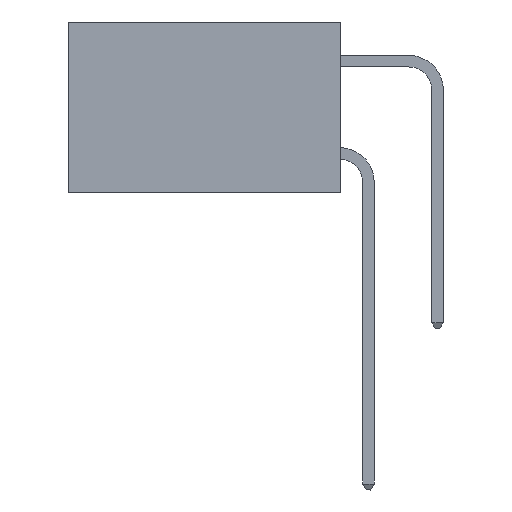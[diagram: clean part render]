
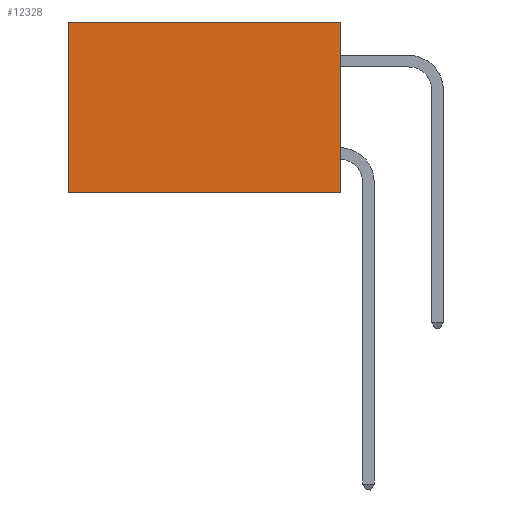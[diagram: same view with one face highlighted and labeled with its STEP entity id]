
A CAD part, left-side view. The second image highlights one B-rep face of the part: STEP entity #12328.
In plain terms, the highlighted planar face has unit normal (-1, 0, 0).
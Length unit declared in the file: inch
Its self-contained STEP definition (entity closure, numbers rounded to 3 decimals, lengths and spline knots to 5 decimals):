
#655 = CARTESIAN_POINT ( 'NONE',  ( 0.277, 0., -0.37 ) ) ;
#1379 = CARTESIAN_POINT ( 'NONE',  ( 0.277, 0.59, -0.37 ) ) ;
#1559 = ORIENTED_EDGE ( 'NONE', *, *, #17714, .T. ) ;
#2286 = CARTESIAN_POINT ( 'NONE',  ( 0.277, 0., -0.37 ) ) ;
#2290 = DIRECTION ( 'NONE',  ( 0., 1., 0. ) ) ;
#3867 = CARTESIAN_POINT ( 'NONE',  ( 0.277, 0.59, 0. ) ) ;
#3962 = ORIENTED_EDGE ( 'NONE', *, *, #21721, .F. ) ;
#6722 = DIRECTION ( 'NONE',  ( 0., 1., 0. ) ) ;
#7480 = DIRECTION ( 'NONE',  ( 1., 0., 0. ) ) ;
#8168 = VERTEX_POINT ( 'NONE', #24331 ) ;
#8585 = CARTESIAN_POINT ( 'NONE',  ( 0.277, 0.59, -0.37 ) ) ;
#8975 = LINE ( 'NONE', #20371, #14972 ) ;
#8997 = LINE ( 'NONE', #9923, #14288 ) ;
#9488 = EDGE_LOOP ( 'NONE', ( #25328, #16363, #3962, #1559 ) ) ;
#9923 = CARTESIAN_POINT ( 'NONE',  ( 0.277, 0., -0.37 ) ) ;
#10253 = LINE ( 'NONE', #1379, #27987 ) ;
#12177 = DIRECTION ( 'NONE',  ( 0., 0., -1. ) ) ;
#12328 = ADVANCED_FACE ( 'NONE', ( #15314 ), #14216, .F. ) ;
#12807 = EDGE_CURVE ( 'NONE', #14659, #15869, #8975, .T. ) ;
#14216 = PLANE ( 'NONE',  #24393 ) ;
#14288 = VECTOR ( 'NONE', #12177, 39.37008 ) ;
#14659 = VERTEX_POINT ( 'NONE', #2286 ) ;
#14972 = VECTOR ( 'NONE', #2290, 39.37008 ) ;
#15052 = EDGE_CURVE ( 'NONE', #17003, #15869, #10253, .T. ) ;
#15314 = FACE_OUTER_BOUND ( 'NONE', #9488, .T. ) ;
#15869 = VERTEX_POINT ( 'NONE', #8585 ) ;
#16363 = ORIENTED_EDGE ( 'NONE', *, *, #12807, .F. ) ;
#17003 = VERTEX_POINT ( 'NONE', #3867 ) ;
#17714 = EDGE_CURVE ( 'NONE', #8168, #17003, #20807, .T. ) ;
#19453 = DIRECTION ( 'NONE',  ( 0., 0., -1. ) ) ;
#20116 = VECTOR ( 'NONE', #6722, 39.37008 ) ;
#20371 = CARTESIAN_POINT ( 'NONE',  ( 0.277, 0., -0.37 ) ) ;
#20807 = LINE ( 'NONE', #28932, #20116 ) ;
#21721 = EDGE_CURVE ( 'NONE', #8168, #14659, #8997, .T. ) ;
#23162 = DIRECTION ( 'NONE',  ( 0., 0., -1. ) ) ;
#24331 = CARTESIAN_POINT ( 'NONE',  ( 0.277, 0., 0. ) ) ;
#24393 = AXIS2_PLACEMENT_3D ( 'NONE', #655, #7480, #23162 ) ;
#25328 = ORIENTED_EDGE ( 'NONE', *, *, #15052, .T. ) ;
#27987 = VECTOR ( 'NONE', #19453, 39.37008 ) ;
#28932 = CARTESIAN_POINT ( 'NONE',  ( 0.277, 0., 0. ) ) ;
